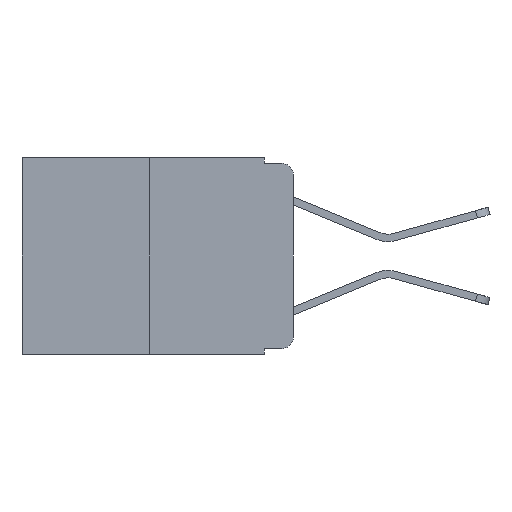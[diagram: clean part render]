
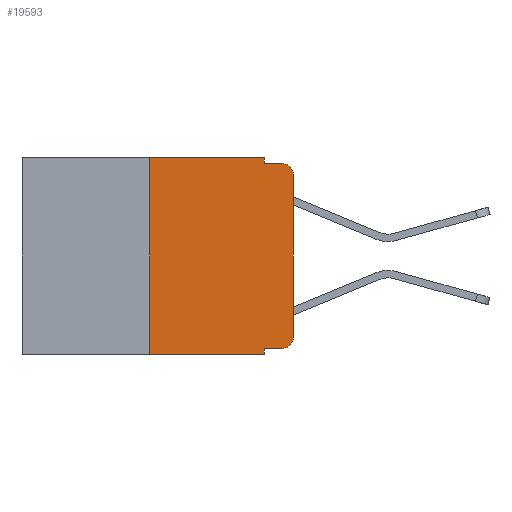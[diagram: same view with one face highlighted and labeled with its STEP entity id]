
A CAD part, left-side view. The second image highlights one B-rep face of the part: STEP entity #19593.
In plain terms, the highlighted planar face has unit normal (-1, 0, 0).
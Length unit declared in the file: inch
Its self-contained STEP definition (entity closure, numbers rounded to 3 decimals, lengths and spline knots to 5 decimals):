
#491 = ORIENTED_EDGE ( 'NONE', *, *, #3908, .F. ) ;
#813 = EDGE_CURVE ( 'NONE', #15787, #8478, #22710, .T. ) ;
#1445 = VECTOR ( 'NONE', #15210, 39.37008 ) ;
#1526 = CARTESIAN_POINT ( 'NONE',  ( 0., 0.051, 0. ) ) ;
#1726 = CARTESIAN_POINT ( 'NONE',  ( 0., 0., -0.03 ) ) ;
#2433 = EDGE_CURVE ( 'NONE', #23839, #9911, #17273, .T. ) ;
#2615 = EDGE_CURVE ( 'NONE', #8478, #5836, #21789, .T. ) ;
#2666 = ORIENTED_EDGE ( 'NONE', *, *, #2433, .T. ) ;
#2984 = AXIS2_PLACEMENT_3D ( 'NONE', #18374, #18325, #16460 ) ;
#3369 = DIRECTION ( 'NONE',  ( 0., -1., 0. ) ) ;
#3475 = DIRECTION ( 'NONE',  ( 0., 0., -1. ) ) ;
#3908 = EDGE_CURVE ( 'NONE', #23839, #17090, #18048, .T. ) ;
#4341 = CARTESIAN_POINT ( 'NONE',  ( 0., 0.02, -0.03 ) ) ;
#4812 = CARTESIAN_POINT ( 'NONE',  ( 0., 0.473, 0. ) ) ;
#4893 = DIRECTION ( 'NONE',  ( 0., 0., -1. ) ) ;
#4956 = ORIENTED_EDGE ( 'NONE', *, *, #21711, .F. ) ;
#5292 = EDGE_CURVE ( 'NONE', #17090, #14926, #7732, .T. ) ;
#5836 = VERTEX_POINT ( 'NONE', #1726 ) ;
#6279 = DIRECTION ( 'NONE',  ( 0., 0., -1. ) ) ;
#6391 = VERTEX_POINT ( 'NONE', #13710 ) ;
#7081 = LINE ( 'NONE', #1526, #12015 ) ;
#7296 = CARTESIAN_POINT ( 'NONE',  ( 0., 0.25, 0. ) ) ;
#7732 = LINE ( 'NONE', #10884, #21761 ) ;
#7762 = EDGE_CURVE ( 'NONE', #5836, #6391, #9671, .T. ) ;
#7891 = AXIS2_PLACEMENT_3D ( 'NONE', #4341, #17344, #6279 ) ;
#8454 = CARTESIAN_POINT ( 'NONE',  ( 0., 0.051, 0. ) ) ;
#8478 = VERTEX_POINT ( 'NONE', #19345 ) ;
#8796 = VECTOR ( 'NONE', #10320, 39.37008 ) ;
#9031 = ORIENTED_EDGE ( 'NONE', *, *, #18832, .F. ) ;
#9137 = LINE ( 'NONE', #21395, #18296 ) ;
#9378 = LINE ( 'NONE', #8454, #8796 ) ;
#9671 = CIRCLE ( 'NONE', #7891, 0.02 ) ;
#9911 = VERTEX_POINT ( 'NONE', #17720 ) ;
#9961 = ORIENTED_EDGE ( 'NONE', *, *, #17620, .F. ) ;
#10320 = DIRECTION ( 'NONE',  ( 0., 0., -1. ) ) ;
#10875 = CARTESIAN_POINT ( 'NONE',  ( 0., 0.25, -0.343 ) ) ;
#10884 = CARTESIAN_POINT ( 'NONE',  ( 0., 0.473, 0. ) ) ;
#11012 = CARTESIAN_POINT ( 'NONE',  ( 0., 0., 0. ) ) ;
#11104 = AXIS2_PLACEMENT_3D ( 'NONE', #4812, #16059, #4893 ) ;
#11511 = ORIENTED_EDGE ( 'NONE', *, *, #5292, .F. ) ;
#11962 = CARTESIAN_POINT ( 'NONE',  ( 0., 0.051, 0. ) ) ;
#12015 = VECTOR ( 'NONE', #3475, 39.37008 ) ;
#12364 = PLANE ( 'NONE',  #11104 ) ;
#12894 = DIRECTION ( 'NONE',  ( 0., 0., 1. ) ) ;
#13136 = CARTESIAN_POINT ( 'NONE',  ( 0., 0.25, 0. ) ) ;
#13215 = VECTOR ( 'NONE', #12894, 39.37008 ) ;
#13536 = VECTOR ( 'NONE', #3369, 39.37008 ) ;
#13710 = CARTESIAN_POINT ( 'NONE',  ( 0., 0.02, -0.01 ) ) ;
#14648 = CARTESIAN_POINT ( 'NONE',  ( 0., 0.051, -0.01 ) ) ;
#14926 = VERTEX_POINT ( 'NONE', #11962 ) ;
#15210 = DIRECTION ( 'NONE',  ( 0., 0., 1. ) ) ;
#15787 = VERTEX_POINT ( 'NONE', #19196 ) ;
#15963 = DIRECTION ( 'NONE',  ( 0., -1., 0. ) ) ;
#16059 = DIRECTION ( 'NONE',  ( 1., 0., 0. ) ) ;
#16168 = CARTESIAN_POINT ( 'NONE',  ( 0., 0.051, -0.01 ) ) ;
#16429 = EDGE_CURVE ( 'NONE', #21897, #15787, #9137, .T. ) ;
#16460 = DIRECTION ( 'NONE',  ( 0., 0., -1. ) ) ;
#16648 = DIRECTION ( 'NONE',  ( 0., -1., 0. ) ) ;
#16729 = ORIENTED_EDGE ( 'NONE', *, *, #7762, .T. ) ;
#16914 = CARTESIAN_POINT ( 'NONE',  ( 0., 0.051, -0.333 ) ) ;
#17090 = VERTEX_POINT ( 'NONE', #13136 ) ;
#17273 = LINE ( 'NONE', #20811, #19803 ) ;
#17344 = DIRECTION ( 'NONE',  ( -1., 0., 0. ) ) ;
#17620 = EDGE_CURVE ( 'NONE', #14926, #21018, #7081, .T. ) ;
#17720 = CARTESIAN_POINT ( 'NONE',  ( 0., 0.051, -0.343 ) ) ;
#18048 = LINE ( 'NONE', #7296, #13215 ) ;
#18296 = VECTOR ( 'NONE', #23198, 39.37008 ) ;
#18325 = DIRECTION ( 'NONE',  ( -1., 0., 0. ) ) ;
#18364 = LINE ( 'NONE', #14648, #13536 ) ;
#18374 = CARTESIAN_POINT ( 'NONE',  ( 0., 0.02, -0.313 ) ) ;
#18832 = EDGE_CURVE ( 'NONE', #21897, #9911, #9378, .T. ) ;
#19196 = CARTESIAN_POINT ( 'NONE',  ( 0., 0.02, -0.333 ) ) ;
#19345 = CARTESIAN_POINT ( 'NONE',  ( 0., 0., -0.313 ) ) ;
#19593 = ADVANCED_FACE ( 'NONE', ( #20161 ), #12364, .F. ) ;
#19803 = VECTOR ( 'NONE', #15963, 39.37008 ) ;
#20161 = FACE_OUTER_BOUND ( 'NONE', #23983, .T. ) ;
#20811 = CARTESIAN_POINT ( 'NONE',  ( 0., 0.473, -0.343 ) ) ;
#21018 = VERTEX_POINT ( 'NONE', #16168 ) ;
#21206 = ORIENTED_EDGE ( 'NONE', *, *, #2615, .T. ) ;
#21395 = CARTESIAN_POINT ( 'NONE',  ( 0., 0.051, -0.333 ) ) ;
#21711 = EDGE_CURVE ( 'NONE', #21018, #6391, #18364, .T. ) ;
#21761 = VECTOR ( 'NONE', #16648, 39.37008 ) ;
#21789 = LINE ( 'NONE', #11012, #1445 ) ;
#21897 = VERTEX_POINT ( 'NONE', #16914 ) ;
#22366 = ORIENTED_EDGE ( 'NONE', *, *, #16429, .T. ) ;
#22710 = CIRCLE ( 'NONE', #2984, 0.02 ) ;
#23198 = DIRECTION ( 'NONE',  ( 0., -1., 0. ) ) ;
#23693 = ORIENTED_EDGE ( 'NONE', *, *, #813, .T. ) ;
#23839 = VERTEX_POINT ( 'NONE', #10875 ) ;
#23983 = EDGE_LOOP ( 'NONE', ( #21206, #16729, #4956, #9961, #11511, #491, #2666, #9031, #22366, #23693 ) ) ;
